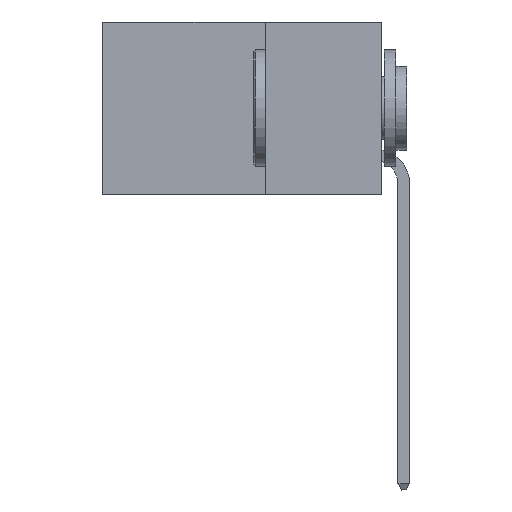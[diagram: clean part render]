
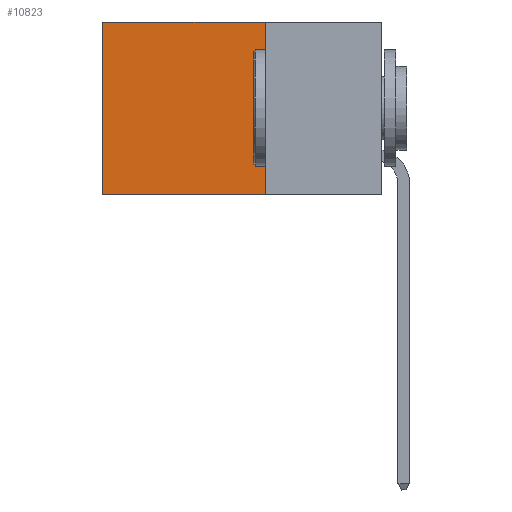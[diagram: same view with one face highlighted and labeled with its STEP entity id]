
A CAD part, left-side view. The second image highlights one B-rep face of the part: STEP entity #10823.
In plain terms, the highlighted planar face has unit normal (-1, 0, 0).
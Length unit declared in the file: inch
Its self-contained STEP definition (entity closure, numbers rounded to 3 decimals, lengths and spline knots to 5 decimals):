
#2128 = PLANE ( 'NONE',  #23082 ) ;
#2839 = CARTESIAN_POINT ( 'NONE',  ( 0.2875, 0.25, -0.37 ) ) ;
#2920 = CARTESIAN_POINT ( 'NONE',  ( 0.2875, 0.25, 0. ) ) ;
#3237 = VECTOR ( 'NONE', #34114, 39.37008 ) ;
#4228 = VERTEX_POINT ( 'NONE', #13997 ) ;
#5985 = CARTESIAN_POINT ( 'NONE',  ( 0.2875, 0.25, 0. ) ) ;
#7163 = EDGE_CURVE ( 'NONE', #12905, #27933, #35047, .T. ) ;
#9332 = LINE ( 'NONE', #28480, #22560 ) ;
#10756 = DIRECTION ( 'NONE',  ( 0., 1., 0. ) ) ;
#10823 = ADVANCED_FACE ( 'NONE', ( #14679 ), #2128, .F. ) ;
#11478 = CARTESIAN_POINT ( 'NONE',  ( 0.2875, 0.25, 0. ) ) ;
#11999 = CARTESIAN_POINT ( 'NONE',  ( 0.2875, 0.25, 0. ) ) ;
#12905 = VERTEX_POINT ( 'NONE', #2920 ) ;
#13046 = LINE ( 'NONE', #44907, #27360 ) ;
#13997 = CARTESIAN_POINT ( 'NONE',  ( 0.2875, 0.6, -0.37 ) ) ;
#14679 = FACE_OUTER_BOUND ( 'NONE', #29605, .T. ) ;
#15152 = EDGE_CURVE ( 'NONE', #12905, #37263, #15708, .T. ) ;
#15708 = LINE ( 'NONE', #11999, #42075 ) ;
#20924 = DIRECTION ( 'NONE',  ( 0., 0., -1. ) ) ;
#22560 = VECTOR ( 'NONE', #20924, 39.37008 ) ;
#23082 = AXIS2_PLACEMENT_3D ( 'NONE', #5985, #44337, #30145 ) ;
#25482 = EDGE_CURVE ( 'NONE', #27933, #4228, #13046, .T. ) ;
#26003 = ORIENTED_EDGE ( 'NONE', *, *, #7163, .F. ) ;
#27360 = VECTOR ( 'NONE', #10756, 39.37008 ) ;
#27933 = VERTEX_POINT ( 'NONE', #2839 ) ;
#28480 = CARTESIAN_POINT ( 'NONE',  ( 0.2875, 0.6, 0. ) ) ;
#29605 = EDGE_LOOP ( 'NONE', ( #39449, #44100, #26003, #38013 ) ) ;
#30145 = DIRECTION ( 'NONE',  ( 0., 0., -1. ) ) ;
#31447 = DIRECTION ( 'NONE',  ( 0., 1., 0. ) ) ;
#33580 = CARTESIAN_POINT ( 'NONE',  ( 0.2875, 0.6, 0. ) ) ;
#34114 = DIRECTION ( 'NONE',  ( 0., 0., -1. ) ) ;
#35047 = LINE ( 'NONE', #11478, #3237 ) ;
#37263 = VERTEX_POINT ( 'NONE', #33580 ) ;
#38013 = ORIENTED_EDGE ( 'NONE', *, *, #15152, .T. ) ;
#38128 = EDGE_CURVE ( 'NONE', #37263, #4228, #9332, .T. ) ;
#39449 = ORIENTED_EDGE ( 'NONE', *, *, #38128, .T. ) ;
#42075 = VECTOR ( 'NONE', #31447, 39.37008 ) ;
#44100 = ORIENTED_EDGE ( 'NONE', *, *, #25482, .F. ) ;
#44337 = DIRECTION ( 'NONE',  ( 1., 0., 0. ) ) ;
#44907 = CARTESIAN_POINT ( 'NONE',  ( 0.2875, 0.25, -0.37 ) ) ;
